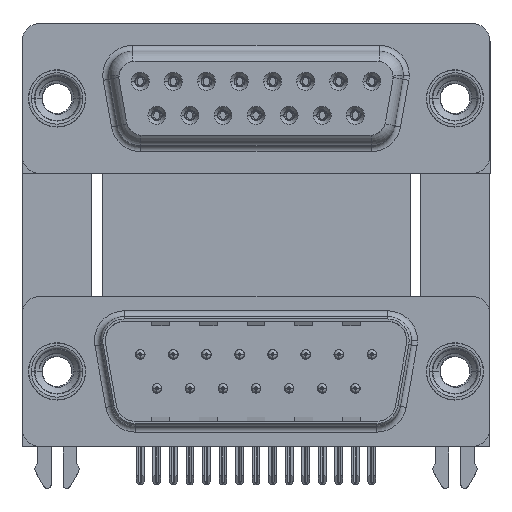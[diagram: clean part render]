
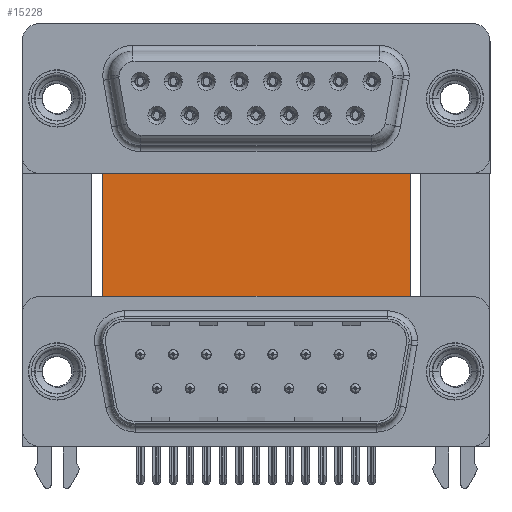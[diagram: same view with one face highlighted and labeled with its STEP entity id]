
A CAD part, top view. The second image highlights one B-rep face of the part: STEP entity #15228.
In plain terms, the highlighted planar face has unit normal (0, 0, 1).
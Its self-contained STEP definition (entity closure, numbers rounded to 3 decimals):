
#20 = AXIS2_PLACEMENT_3D ( 'NONE', #42015, #31156, #20759 ) ;
#1560 = EDGE_CURVE ( 'NONE', #6424, #44442, #11604, .T. ) ;
#1857 = CARTESIAN_POINT ( 'NONE',  ( 29.58, 16.585, -12. ) ) ;
#4516 = DIRECTION ( 'NONE',  ( 1., 0., 0. ) ) ;
#5627 = VECTOR ( 'NONE', #28393, 1000. ) ;
#6190 = LINE ( 'NONE', #41619, #17053 ) ;
#6203 = CARTESIAN_POINT ( 'NONE',  ( 3.79, 16.585, -12. ) ) ;
#6424 = VERTEX_POINT ( 'NONE', #10918 ) ;
#9500 = DIRECTION ( 'NONE',  ( 1., 0., 0. ) ) ;
#10918 = CARTESIAN_POINT ( 'NONE',  ( 3.79, -3.735, -12. ) ) ;
#11604 = LINE ( 'NONE', #18225, #38564 ) ;
#14371 = CARTESIAN_POINT ( 'NONE',  ( 3.79, 16.585, -12. ) ) ;
#15228 = ADVANCED_FACE ( 'NONE', ( #45546 ), #16278, .F. ) ;
#16018 = DIRECTION ( 'NONE',  ( 0., -1., 0. ) ) ;
#16278 = PLANE ( 'NONE',  #20 ) ;
#17053 = VECTOR ( 'NONE', #9500, 1000. ) ;
#17394 = EDGE_CURVE ( 'NONE', #29182, #44442, #33962, .T. ) ;
#18225 = CARTESIAN_POINT ( 'NONE',  ( 3.79, -3.735, -12. ) ) ;
#20759 = DIRECTION ( 'NONE',  ( -1., 0., 0. ) ) ;
#21572 = CARTESIAN_POINT ( 'NONE',  ( 29.58, -3.735, -12. ) ) ;
#23620 = ORIENTED_EDGE ( 'NONE', *, *, #17394, .F. ) ;
#28374 = ORIENTED_EDGE ( 'NONE', *, *, #33532, .F. ) ;
#28393 = DIRECTION ( 'NONE',  ( 0., -1., 0. ) ) ;
#29085 = CARTESIAN_POINT ( 'NONE',  ( 29.58, 16.585, -12. ) ) ;
#29182 = VERTEX_POINT ( 'NONE', #29085 ) ;
#31156 = DIRECTION ( 'NONE',  ( 0., 0., -1. ) ) ;
#32869 = EDGE_LOOP ( 'NONE', ( #46528, #23620, #28374, #34385 ) ) ;
#33133 = VECTOR ( 'NONE', #16018, 1000. ) ;
#33532 = EDGE_CURVE ( 'NONE', #45493, #29182, #6190, .T. ) ;
#33962 = LINE ( 'NONE', #1857, #33133 ) ;
#34385 = ORIENTED_EDGE ( 'NONE', *, *, #44841, .T. ) ;
#38564 = VECTOR ( 'NONE', #4516, 1000. ) ;
#39250 = LINE ( 'NONE', #6203, #5627 ) ;
#41619 = CARTESIAN_POINT ( 'NONE',  ( 3.79, 16.585, -12. ) ) ;
#42015 = CARTESIAN_POINT ( 'NONE',  ( 3.79, 16.585, -12. ) ) ;
#44442 = VERTEX_POINT ( 'NONE', #21572 ) ;
#44841 = EDGE_CURVE ( 'NONE', #45493, #6424, #39250, .T. ) ;
#45493 = VERTEX_POINT ( 'NONE', #14371 ) ;
#45546 = FACE_OUTER_BOUND ( 'NONE', #32869, .T. ) ;
#46528 = ORIENTED_EDGE ( 'NONE', *, *, #1560, .T. ) ;
